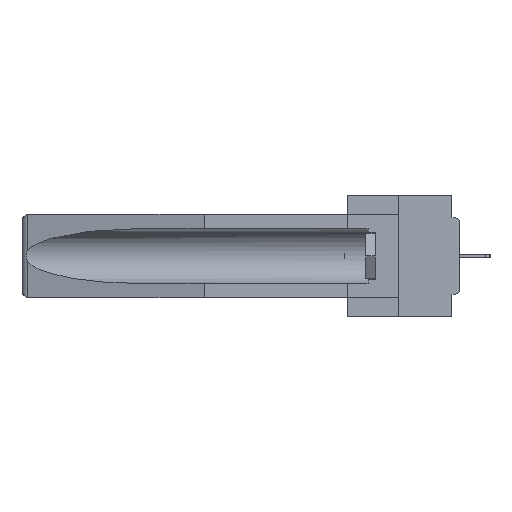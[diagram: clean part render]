
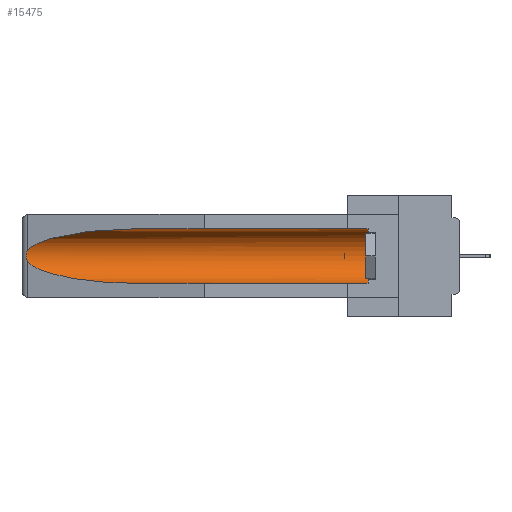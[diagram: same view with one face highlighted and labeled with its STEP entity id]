
A CAD part, left-side view. The second image highlights one B-rep face of the part: STEP entity #15475.
In plain terms, the highlighted cylindrical face has radius 2.857 mm (diameter 5.715 mm), a partial arc.
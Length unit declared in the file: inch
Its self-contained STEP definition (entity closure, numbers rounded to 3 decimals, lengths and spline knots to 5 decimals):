
#426 = CARTESIAN_POINT ( 'NONE',  ( 0.155, 1.07973, -0.284 ) ) ;
#1634 = DIRECTION ( 'NONE',  ( 0., 1., 0. ) ) ;
#2254 = VERTEX_POINT ( 'NONE', #426 ) ;
#3101 = CARTESIAN_POINT ( 'NONE',  ( 0.26537, 1.52718, -0.19328 ) ) ;
#3254 = DIRECTION ( 'NONE',  ( 0., 0., 1. ) ) ;
#3341 = ORIENTED_EDGE ( 'NONE', *, *, #41921, .F. ) ;
#3913 = ORIENTED_EDGE ( 'NONE', *, *, #9220, .T. ) ;
#5017 = B_SPLINE_CURVE_WITH_KNOTS ( 'NONE', 3,
 ( #9635, #32451, #12965, #35649, #16222, #38919, #19476, #42174, #22772, #3101 ),
 .UNSPECIFIED., .F., .F.,
 ( 4, 2, 2, 2, 4 ),
 ( 0., 0.00029, 0.00058, 0.00087, 0.00117 ),
 .UNSPECIFIED. ) ;
#5537 = AXIS2_PLACEMENT_3D ( 'NONE', #19499, #22941, #3254 ) ;
#6838 = CARTESIAN_POINT ( 'NONE',  ( 0.155, 1.07973, -0.059 ) ) ;
#8280 = EDGE_CURVE ( 'NONE', #20582, #33025, #24707, .T. ) ;
#9060 = ORIENTED_EDGE ( 'NONE', *, *, #11008, .T. ) ;
#9220 = EDGE_CURVE ( 'NONE', #41159, #20582, #40701, .T. ) ;
#9635 = CARTESIAN_POINT ( 'NONE',  ( 0.26537, 1.52718, -0.14972 ) ) ;
#9952 = DIRECTION ( 'NONE',  ( 0., 1., 0. ) ) ;
#10163 = CARTESIAN_POINT ( 'NONE',  ( 0.26537, 1.52718, -0.14972 ) ) ;
#10616 = ORIENTED_EDGE ( 'NONE', *, *, #8280, .T. ) ;
#11007 = DIRECTION ( 'NONE',  ( 0., -1., 0. ) ) ;
#11008 = EDGE_CURVE ( 'NONE', #35215, #2254, #32264, .T. ) ;
#11697 = ORIENTED_EDGE ( 'NONE', *, *, #15034, .T. ) ;
#12676 = CARTESIAN_POINT ( 'NONE',  ( 0.21114, 1.30732, -0.284 ) ) ;
#12838 = EDGE_CURVE ( 'NONE', #33025, #35215, #5017, .T. ) ;
#12965 = CARTESIAN_POINT ( 'NONE',  ( 0.26654, 1.53092, -0.15636 ) ) ;
#13849 = LINE ( 'NONE', #29496, #15896 ) ;
#15034 = EDGE_CURVE ( 'NONE', #36883, #41159, #15877, .T. ) ;
#15475 = ADVANCED_FACE ( 'NONE', ( #28538 ), #18819, .F. ) ;
#15799 = CARTESIAN_POINT ( 'NONE',  ( 0.25451, 1.48313, -0.24835 ) ) ;
#15877 = CIRCLE ( 'NONE', #26919, 0.1125 ) ;
#15896 = VECTOR ( 'NONE', #9952, 39.37008 ) ;
#16222 = CARTESIAN_POINT ( 'NONE',  ( 0.2675, 1.53308, -0.16763 ) ) ;
#18819 = CYLINDRICAL_SURFACE ( 'NONE', #5537, 0.1125 ) ;
#19476 = CARTESIAN_POINT ( 'NONE',  ( 0.2673, 1.53269, -0.17917 ) ) ;
#19499 = CARTESIAN_POINT ( 'NONE',  ( 0.155, -0.30754, -0.1715 ) ) ;
#19852 = CARTESIAN_POINT ( 'NONE',  ( 0.21114, 1.30732, -0.059 ) ) ;
#19867 = CARTESIAN_POINT ( 'NONE',  ( 0.155, 0.126, -0.059 ) ) ;
#20582 = VERTEX_POINT ( 'NONE', #21615 ) ;
#21615 = CARTESIAN_POINT ( 'NONE',  ( 0.155, 1.07973, -0.059 ) ) ;
#22772 = CARTESIAN_POINT ( 'NONE',  ( 0.26597, 1.5296, -0.19026 ) ) ;
#22941 = DIRECTION ( 'NONE',  ( 0., 1., 0. ) ) ;
#22965 = EDGE_LOOP ( 'NONE', ( #10616, #24405, #9060, #3341, #11697, #3913 ) ) ;
#23161 = CARTESIAN_POINT ( 'NONE',  ( 0.25451, 1.48313, -0.09465 ) ) ;
#23470 = VECTOR ( 'NONE', #1634, 39.37008 ) ;
#24405 = ORIENTED_EDGE ( 'NONE', *, *, #12838, .T. ) ;
#24707 =( BOUNDED_CURVE ( )  B_SPLINE_CURVE ( 3, ( #6838, #19852, #23161, #10163 ),
 .UNSPECIFIED., .F., .F. ) 
 B_SPLINE_CURVE_WITH_KNOTS ( ( 4, 4 ),
 ( 4.71239, 6.08839 ),
 .UNSPECIFIED. ) 
 CURVE ( )  GEOMETRIC_REPRESENTATION_ITEM ( )  RATIONAL_B_SPLINE_CURVE ( ( 1., 0.848, 0.848, 1. ) ) 
 REPRESENTATION_ITEM ( '' )  );
#26919 = AXIS2_PLACEMENT_3D ( 'NONE', #30517, #11007, #33769 ) ;
#28538 = FACE_OUTER_BOUND ( 'NONE', #22965, .T. ) ;
#28755 = CARTESIAN_POINT ( 'NONE',  ( 0.26537, 1.52718, -0.19328 ) ) ;
#29496 = CARTESIAN_POINT ( 'NONE',  ( 0.155, -0.30754, -0.284 ) ) ;
#29620 = CARTESIAN_POINT ( 'NONE',  ( 0.155, 0.126, -0.284 ) ) ;
#30517 = CARTESIAN_POINT ( 'NONE',  ( 0.155, 0.126, -0.1715 ) ) ;
#31069 = CARTESIAN_POINT ( 'NONE',  ( 0.26537, 1.52718, -0.19328 ) ) ;
#31176 = CARTESIAN_POINT ( 'NONE',  ( 0.155, -0.30754, -0.059 ) ) ;
#32151 = CARTESIAN_POINT ( 'NONE',  ( 0.26537, 1.52718, -0.14972 ) ) ;
#32264 =( BOUNDED_CURVE ( )  B_SPLINE_CURVE ( 3, ( #28755, #15799, #12676, #35365 ),
 .UNSPECIFIED., .F., .T. ) 
 B_SPLINE_CURVE_WITH_KNOTS ( ( 4, 4 ),
 ( 0.1948, 1.5708 ),
 .UNSPECIFIED. ) 
 CURVE ( )  GEOMETRIC_REPRESENTATION_ITEM ( )  RATIONAL_B_SPLINE_CURVE ( ( 1., 0.848, 0.848, 1. ) ) 
 REPRESENTATION_ITEM ( '' )  );
#32451 = CARTESIAN_POINT ( 'NONE',  ( 0.26597, 1.52961, -0.15275 ) ) ;
#33025 = VERTEX_POINT ( 'NONE', #32151 ) ;
#33769 = DIRECTION ( 'NONE',  ( 0., 0., 1. ) ) ;
#35215 = VERTEX_POINT ( 'NONE', #31069 ) ;
#35365 = CARTESIAN_POINT ( 'NONE',  ( 0.155, 1.07973, -0.284 ) ) ;
#35649 = CARTESIAN_POINT ( 'NONE',  ( 0.2673, 1.5327, -0.16383 ) ) ;
#36883 = VERTEX_POINT ( 'NONE', #29620 ) ;
#38919 = CARTESIAN_POINT ( 'NONE',  ( 0.2675, 1.53308, -0.17534 ) ) ;
#40701 = LINE ( 'NONE', #31176, #23470 ) ;
#41159 = VERTEX_POINT ( 'NONE', #19867 ) ;
#41921 = EDGE_CURVE ( 'NONE', #36883, #2254, #13849, .T. ) ;
#42174 = CARTESIAN_POINT ( 'NONE',  ( 0.26655, 1.53094, -0.18657 ) ) ;
